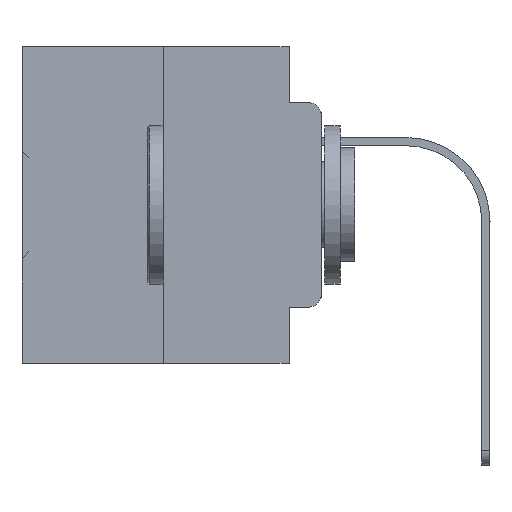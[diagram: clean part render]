
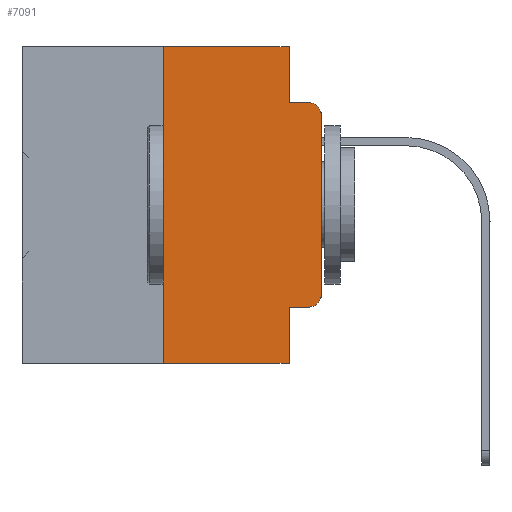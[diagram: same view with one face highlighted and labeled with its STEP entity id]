
A CAD part, left-side view. The second image highlights one B-rep face of the part: STEP entity #7091.
In plain terms, the highlighted planar face has unit normal (-1, 0, 0).
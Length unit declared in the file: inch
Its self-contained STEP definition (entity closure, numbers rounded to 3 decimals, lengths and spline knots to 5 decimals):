
#438 = ORIENTED_EDGE ( 'NONE', *, *, #26751, .T. ) ;
#1423 = DIRECTION ( 'NONE',  ( 0., -1., 0. ) ) ;
#1497 = DIRECTION ( 'NONE',  ( 0., 0., -1. ) ) ;
#1511 = CARTESIAN_POINT ( 'NONE',  ( 0., 0.02, -0.0885 ) ) ;
#1909 = CARTESIAN_POINT ( 'NONE',  ( 0., 0.051, -0.4115 ) ) ;
#2949 = LINE ( 'NONE', #14432, #12625 ) ;
#3598 = VECTOR ( 'NONE', #25127, 39.37008 ) ;
#4202 = VECTOR ( 'NONE', #1423, 39.37008 ) ;
#4270 = VECTOR ( 'NONE', #32155, 39.37008 ) ;
#4555 = CARTESIAN_POINT ( 'NONE',  ( 0., 0.051, -0.4115 ) ) ;
#4609 = ORIENTED_EDGE ( 'NONE', *, *, #16920, .F. ) ;
#4857 = CARTESIAN_POINT ( 'NONE',  ( 0., 0.051, -0.0885 ) ) ;
#5021 = VERTEX_POINT ( 'NONE', #27912 ) ;
#5764 = DIRECTION ( 'NONE',  ( -1., 0., 0. ) ) ;
#5911 = AXIS2_PLACEMENT_3D ( 'NONE', #24302, #10220, #33151 ) ;
#6795 = LINE ( 'NONE', #20712, #4270 ) ;
#7091 = ADVANCED_FACE ( 'NONE', ( #23881 ), #15812, .F. ) ;
#8303 = ORIENTED_EDGE ( 'NONE', *, *, #15673, .T. ) ;
#8764 = VERTEX_POINT ( 'NONE', #4555 ) ;
#9872 = VERTEX_POINT ( 'NONE', #34127 ) ;
#10220 = DIRECTION ( 'NONE',  ( -1., 0., 0. ) ) ;
#10299 = LINE ( 'NONE', #21772, #17333 ) ;
#10325 = EDGE_CURVE ( 'NONE', #8764, #27956, #6795, .T. ) ;
#10461 = LINE ( 'NONE', #33397, #28815 ) ;
#10627 = LINE ( 'NONE', #22102, #4202 ) ;
#10939 = VERTEX_POINT ( 'NONE', #4857 ) ;
#11429 = LINE ( 'NONE', #1909, #37013 ) ;
#12625 = VECTOR ( 'NONE', #14228, 39.37008 ) ;
#14228 = DIRECTION ( 'NONE',  ( 0., -1., 0. ) ) ;
#14432 = CARTESIAN_POINT ( 'NONE',  ( 0., 0.473, -0.5 ) ) ;
#15376 = EDGE_CURVE ( 'NONE', #9872, #22269, #10299, .T. ) ;
#15673 = EDGE_CURVE ( 'NONE', #22922, #9872, #23935, .T. ) ;
#15812 = PLANE ( 'NONE',  #20099 ) ;
#16221 = CARTESIAN_POINT ( 'NONE',  ( 0., 0.25, 0. ) ) ;
#16920 = EDGE_CURVE ( 'NONE', #18947, #5021, #10627, .T. ) ;
#16974 = ORIENTED_EDGE ( 'NONE', *, *, #24830, .F. ) ;
#17333 = VECTOR ( 'NONE', #30392, 39.37008 ) ;
#17457 = DIRECTION ( 'NONE',  ( 0., 0., -1. ) ) ;
#17948 = VECTOR ( 'NONE', #22530, 39.37008 ) ;
#18936 = CARTESIAN_POINT ( 'NONE',  ( 0., 0.051, -0.0885 ) ) ;
#18947 = VERTEX_POINT ( 'NONE', #16221 ) ;
#20099 = AXIS2_PLACEMENT_3D ( 'NONE', #26899, #27281, #1497 ) ;
#20712 = CARTESIAN_POINT ( 'NONE',  ( 0., 0.051, 0. ) ) ;
#20811 = ORIENTED_EDGE ( 'NONE', *, *, #15376, .T. ) ;
#21645 = VERTEX_POINT ( 'NONE', #1511 ) ;
#21772 = CARTESIAN_POINT ( 'NONE',  ( 0., 0., 0. ) ) ;
#21937 = ORIENTED_EDGE ( 'NONE', *, *, #25799, .F. ) ;
#22102 = CARTESIAN_POINT ( 'NONE',  ( 0., 0.473, 0. ) ) ;
#22269 = VERTEX_POINT ( 'NONE', #31306 ) ;
#22367 = ORIENTED_EDGE ( 'NONE', *, *, #10325, .F. ) ;
#22408 = ORIENTED_EDGE ( 'NONE', *, *, #26672, .T. ) ;
#22530 = DIRECTION ( 'NONE',  ( 0., 0., -1. ) ) ;
#22922 = VERTEX_POINT ( 'NONE', #27482 ) ;
#23881 = FACE_OUTER_BOUND ( 'NONE', #34966, .T. ) ;
#23935 = CIRCLE ( 'NONE', #5911, 0.02 ) ;
#24302 = CARTESIAN_POINT ( 'NONE',  ( 0., 0.02, -0.3915 ) ) ;
#24676 = DIRECTION ( 'NONE',  ( 0., -1., 0. ) ) ;
#24830 = EDGE_CURVE ( 'NONE', #5021, #10939, #25367, .T. ) ;
#25127 = DIRECTION ( 'NONE',  ( 0., -1., 0. ) ) ;
#25367 = LINE ( 'NONE', #28734, #17948 ) ;
#25451 = EDGE_CURVE ( 'NONE', #30230, #27956, #2949, .T. ) ;
#25696 = EDGE_CURVE ( 'NONE', #10939, #21645, #36597, .T. ) ;
#25799 = EDGE_CURVE ( 'NONE', #30230, #18947, #10461, .T. ) ;
#25903 = CARTESIAN_POINT ( 'NONE',  ( 0., 0.02, -0.1085 ) ) ;
#26672 = EDGE_CURVE ( 'NONE', #8764, #22922, #11429, .T. ) ;
#26751 = EDGE_CURVE ( 'NONE', #22269, #21645, #32203, .T. ) ;
#26899 = CARTESIAN_POINT ( 'NONE',  ( 0., 0.473, 0. ) ) ;
#27281 = DIRECTION ( 'NONE',  ( 1., 0., 0. ) ) ;
#27482 = CARTESIAN_POINT ( 'NONE',  ( 0., 0.02, -0.4115 ) ) ;
#27689 = CARTESIAN_POINT ( 'NONE',  ( 0., 0.051, -0.5 ) ) ;
#27912 = CARTESIAN_POINT ( 'NONE',  ( 0., 0.051, 0. ) ) ;
#27956 = VERTEX_POINT ( 'NONE', #27689 ) ;
#28734 = CARTESIAN_POINT ( 'NONE',  ( 0., 0.051, 0. ) ) ;
#28815 = VECTOR ( 'NONE', #30750, 39.37008 ) ;
#30230 = VERTEX_POINT ( 'NONE', #34486 ) ;
#30392 = DIRECTION ( 'NONE',  ( 0., 0., 1. ) ) ;
#30750 = DIRECTION ( 'NONE',  ( 0., 0., 1. ) ) ;
#31306 = CARTESIAN_POINT ( 'NONE',  ( 0., 0., -0.1085 ) ) ;
#32013 = ORIENTED_EDGE ( 'NONE', *, *, #25696, .F. ) ;
#32155 = DIRECTION ( 'NONE',  ( 0., 0., -1. ) ) ;
#32203 = CIRCLE ( 'NONE', #34630, 0.02 ) ;
#33151 = DIRECTION ( 'NONE',  ( 0., 0., -1. ) ) ;
#33397 = CARTESIAN_POINT ( 'NONE',  ( 0., 0.25, 0. ) ) ;
#34127 = CARTESIAN_POINT ( 'NONE',  ( 0., 0., -0.3915 ) ) ;
#34197 = ORIENTED_EDGE ( 'NONE', *, *, #25451, .T. ) ;
#34486 = CARTESIAN_POINT ( 'NONE',  ( 0., 0.25, -0.5 ) ) ;
#34630 = AXIS2_PLACEMENT_3D ( 'NONE', #25903, #5764, #17457 ) ;
#34966 = EDGE_LOOP ( 'NONE', ( #20811, #438, #32013, #16974, #4609, #21937, #34197, #22367, #22408, #8303 ) ) ;
#36597 = LINE ( 'NONE', #18936, #3598 ) ;
#37013 = VECTOR ( 'NONE', #24676, 39.37008 ) ;
